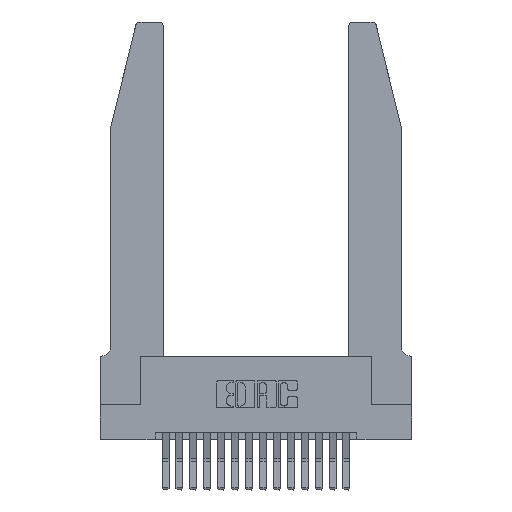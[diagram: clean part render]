
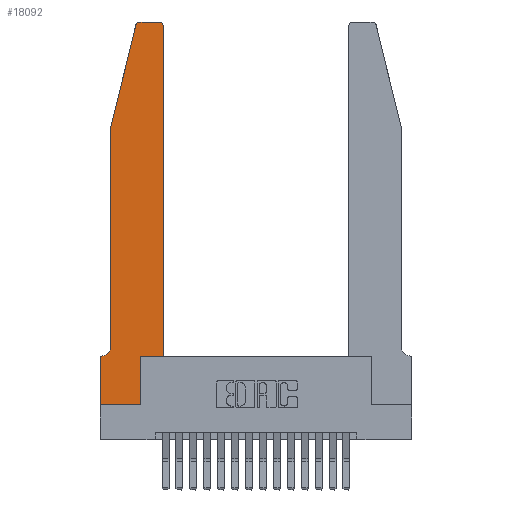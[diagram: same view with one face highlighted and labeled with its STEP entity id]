
A CAD part, top view. The second image highlights one B-rep face of the part: STEP entity #18092.
In plain terms, the highlighted planar face has unit normal (0, 0, 1).
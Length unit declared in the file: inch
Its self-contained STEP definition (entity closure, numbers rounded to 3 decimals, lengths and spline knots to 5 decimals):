
#184 = EDGE_CURVE ( 'NONE', #9467, #12443, #3690, .T. ) ;
#185 = ORIENTED_EDGE ( 'NONE', *, *, #19536, .T. ) ;
#319 = VECTOR ( 'NONE', #1607, 39.37008 ) ;
#493 = CARTESIAN_POINT ( 'NONE',  ( 0., 0.35, 0.37 ) ) ;
#597 = LINE ( 'NONE', #14381, #3597 ) ;
#740 = VERTEX_POINT ( 'NONE', #10141 ) ;
#1325 = CARTESIAN_POINT ( 'NONE',  ( 0.0755, 0.42, 0.37 ) ) ;
#1607 = DIRECTION ( 'NONE',  ( 0., -1., 0. ) ) ;
#1815 = VERTEX_POINT ( 'NONE', #2019 ) ;
#2019 = CARTESIAN_POINT ( 'NONE',  ( 0.4505, 0.35, 0.37 ) ) ;
#2089 = DIRECTION ( 'NONE',  ( 1., 0., 0. ) ) ;
#2964 = CARTESIAN_POINT ( 'NONE',  ( 0., 0.35, 0.37 ) ) ;
#3112 = ORIENTED_EDGE ( 'NONE', *, *, #184, .T. ) ;
#3296 = ORIENTED_EDGE ( 'NONE', *, *, #17924, .T. ) ;
#3396 = CARTESIAN_POINT ( 'NONE',  ( 0.4505, 2.72, 0.37 ) ) ;
#3550 = CARTESIAN_POINT ( 'NONE',  ( 0.0055, 0.42, 0.37 ) ) ;
#3597 = VECTOR ( 'NONE', #14454, 39.37008 ) ;
#3690 = CIRCLE ( 'NONE', #5870, 0.03 ) ;
#3729 = EDGE_CURVE ( 'NONE', #12249, #8609, #597, .T. ) ;
#3949 = DIRECTION ( 'NONE',  ( -1., 0., 0. ) ) ;
#4019 = ORIENTED_EDGE ( 'NONE', *, *, #15292, .T. ) ;
#4203 = LINE ( 'NONE', #7233, #11710 ) ;
#4209 = CARTESIAN_POINT ( 'NONE',  ( 0.284, 2.75, 0.37 ) ) ;
#4437 = CARTESIAN_POINT ( 'NONE',  ( 0.0755, 2., 0.37 ) ) ;
#4515 = LINE ( 'NONE', #9311, #319 ) ;
#4761 = CARTESIAN_POINT ( 'NONE',  ( 0.0055, 0.35, 0.37 ) ) ;
#4927 = DIRECTION ( 'NONE',  ( 0., 0., 1. ) ) ;
#4977 = EDGE_CURVE ( 'NONE', #5185, #9467, #18818, .T. ) ;
#5128 = DIRECTION ( 'NONE',  ( -1., 0., 0. ) ) ;
#5185 = VERTEX_POINT ( 'NONE', #17857 ) ;
#5297 = VECTOR ( 'NONE', #19264, 39.37008 ) ;
#5747 = CARTESIAN_POINT ( 'NONE',  ( 0.0755, 0.35, 0.37 ) ) ;
#5836 = CARTESIAN_POINT ( 'NONE',  ( 0., 0., 0.37 ) ) ;
#5870 = AXIS2_PLACEMENT_3D ( 'NONE', #5885, #14592, #12453 ) ;
#5885 = CARTESIAN_POINT ( 'NONE',  ( 0.284, 2.72, 0.37 ) ) ;
#6290 = DIRECTION ( 'NONE',  ( 0., 1., 0. ) ) ;
#6741 = LINE ( 'NONE', #4437, #18158 ) ;
#7079 = ORIENTED_EDGE ( 'NONE', *, *, #4977, .T. ) ;
#7233 = CARTESIAN_POINT ( 'NONE',  ( 0.4505, 0.35, 0.37 ) ) ;
#7253 = DIRECTION ( 'NONE',  ( -1., 0., 0. ) ) ;
#7761 = VECTOR ( 'NONE', #6290, 39.37008 ) ;
#8112 = EDGE_CURVE ( 'NONE', #8609, #16070, #12158, .T. ) ;
#8115 = CARTESIAN_POINT ( 'NONE',  ( 0., 0., 0.37 ) ) ;
#8130 = PLANE ( 'NONE',  #9196 ) ;
#8365 = ORIENTED_EDGE ( 'NONE', *, *, #3729, .T. ) ;
#8609 = VERTEX_POINT ( 'NONE', #17937 ) ;
#8627 = VERTEX_POINT ( 'NONE', #1325 ) ;
#8746 = DIRECTION ( 'NONE',  ( 0., 1., 0. ) ) ;
#8787 = FACE_OUTER_BOUND ( 'NONE', #17358, .T. ) ;
#9196 = AXIS2_PLACEMENT_3D ( 'NONE', #493, #11181, #2089 ) ;
#9210 = CARTESIAN_POINT ( 'NONE',  ( 0.2865, 0.35, 0.37 ) ) ;
#9311 = CARTESIAN_POINT ( 'NONE',  ( 0.0755, 2., 0.37 ) ) ;
#9467 = VERTEX_POINT ( 'NONE', #4209 ) ;
#9563 = ORIENTED_EDGE ( 'NONE', *, *, #8112, .T. ) ;
#10110 = ORIENTED_EDGE ( 'NONE', *, *, #13455, .T. ) ;
#10141 = CARTESIAN_POINT ( 'NONE',  ( 0.0755, 2., 0.37 ) ) ;
#10821 = VERTEX_POINT ( 'NONE', #3396 ) ;
#11181 = DIRECTION ( 'NONE',  ( 0., 0., 1. ) ) ;
#11498 = VERTEX_POINT ( 'NONE', #4761 ) ;
#11710 = VECTOR ( 'NONE', #8746, 39.37008 ) ;
#11877 = LINE ( 'NONE', #18698, #15441 ) ;
#12158 = LINE ( 'NONE', #12177, #7761 ) ;
#12177 = CARTESIAN_POINT ( 'NONE',  ( 0.2865, 0.35, 0.37 ) ) ;
#12249 = VERTEX_POINT ( 'NONE', #8115 ) ;
#12443 = VERTEX_POINT ( 'NONE', #13034 ) ;
#12453 = DIRECTION ( 'NONE',  ( 1., 0., 0. ) ) ;
#12687 = EDGE_CURVE ( 'NONE', #10821, #5185, #18004, .T. ) ;
#12909 = ORIENTED_EDGE ( 'NONE', *, *, #14737, .T. ) ;
#13034 = CARTESIAN_POINT ( 'NONE',  ( 0.25487, 2.72718, 0.37 ) ) ;
#13386 = DIRECTION ( 'NONE',  ( -0.239, -0.971, 0. ) ) ;
#13455 = EDGE_CURVE ( 'NONE', #16070, #1815, #11877, .T. ) ;
#13692 = VERTEX_POINT ( 'NONE', #2964 ) ;
#13868 = CARTESIAN_POINT ( 'NONE',  ( 0.4205, 2.72, 0.37 ) ) ;
#14065 = DIRECTION ( 'NONE',  ( 0., 0., -1. ) ) ;
#14381 = CARTESIAN_POINT ( 'NONE',  ( 0., 0., 0.37 ) ) ;
#14454 = DIRECTION ( 'NONE',  ( 1., 0., 0. ) ) ;
#14592 = DIRECTION ( 'NONE',  ( 0., 0., 1. ) ) ;
#14737 = EDGE_CURVE ( 'NONE', #12443, #740, #6741, .T. ) ;
#14851 = VECTOR ( 'NONE', #3949, 39.37008 ) ;
#15292 = EDGE_CURVE ( 'NONE', #13692, #12249, #17229, .T. ) ;
#15429 = DIRECTION ( 'NONE',  ( 1., 0., 0. ) ) ;
#15441 = VECTOR ( 'NONE', #17222, 39.37008 ) ;
#16070 = VERTEX_POINT ( 'NONE', #9210 ) ;
#16227 = EDGE_CURVE ( 'NONE', #8627, #11498, #17650, .T. ) ;
#16534 = AXIS2_PLACEMENT_3D ( 'NONE', #13868, #4927, #15429 ) ;
#16690 = VECTOR ( 'NONE', #7253, 39.37008 ) ;
#17113 = ORIENTED_EDGE ( 'NONE', *, *, #16227, .T. ) ;
#17155 = LINE ( 'NONE', #5747, #16690 ) ;
#17222 = DIRECTION ( 'NONE',  ( 1., 0., 0. ) ) ;
#17229 = LINE ( 'NONE', #5836, #5297 ) ;
#17358 = EDGE_LOOP ( 'NONE', ( #7079, #3112, #12909, #3296, #17113, #19301, #4019, #8365, #9563, #10110, #185, #18332 ) ) ;
#17650 = CIRCLE ( 'NONE', #17795, 0.07 ) ;
#17795 = AXIS2_PLACEMENT_3D ( 'NONE', #3550, #14065, #5128 ) ;
#17857 = CARTESIAN_POINT ( 'NONE',  ( 0.4205, 2.75, 0.37 ) ) ;
#17924 = EDGE_CURVE ( 'NONE', #740, #8627, #4515, .T. ) ;
#17937 = CARTESIAN_POINT ( 'NONE',  ( 0.2865, 0., 0.37 ) ) ;
#18004 = CIRCLE ( 'NONE', #16534, 0.03 ) ;
#18092 = ADVANCED_FACE ( 'NONE', ( #8787 ), #8130, .T. ) ;
#18158 = VECTOR ( 'NONE', #13386, 39.37008 ) ;
#18332 = ORIENTED_EDGE ( 'NONE', *, *, #12687, .T. ) ;
#18698 = CARTESIAN_POINT ( 'NONE',  ( 0.4505, 0.35, 0.37 ) ) ;
#18818 = LINE ( 'NONE', #18907, #14851 ) ;
#18907 = CARTESIAN_POINT ( 'NONE',  ( 0.2605, 2.75, 0.37 ) ) ;
#18985 = EDGE_CURVE ( 'NONE', #11498, #13692, #17155, .T. ) ;
#19264 = DIRECTION ( 'NONE',  ( 0., -1., 0. ) ) ;
#19301 = ORIENTED_EDGE ( 'NONE', *, *, #18985, .T. ) ;
#19536 = EDGE_CURVE ( 'NONE', #1815, #10821, #4203, .T. ) ;
